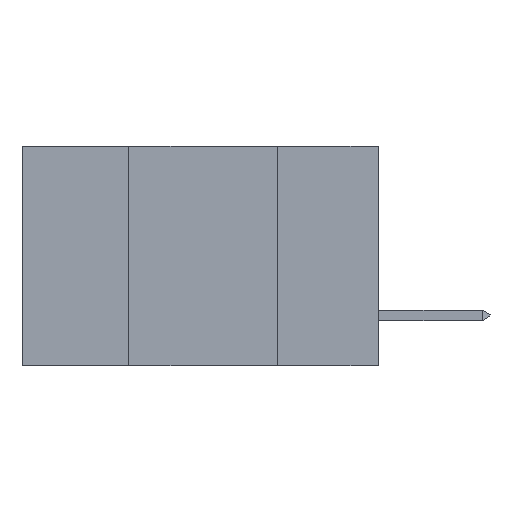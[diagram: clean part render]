
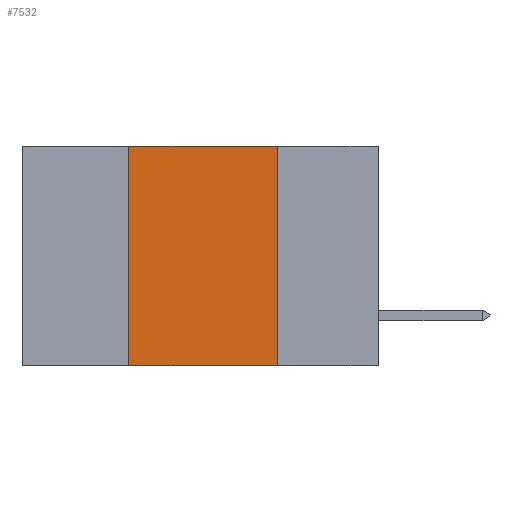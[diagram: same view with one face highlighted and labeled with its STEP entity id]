
A CAD part, left-side view. The second image highlights one B-rep face of the part: STEP entity #7532.
In plain terms, the highlighted planar face has unit normal (-1, 0, 0).
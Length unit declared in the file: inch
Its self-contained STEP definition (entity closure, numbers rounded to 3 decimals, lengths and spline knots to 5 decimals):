
#207 = VECTOR ( 'NONE', #2808, 39.37008 ) ;
#284 = FACE_OUTER_BOUND ( 'NONE', #3619, .T. ) ;
#699 = ORIENTED_EDGE ( 'NONE', *, *, #9616, .F. ) ;
#1013 = CARTESIAN_POINT ( 'NONE',  ( 0., 0.17, -0.37 ) ) ;
#1340 = CARTESIAN_POINT ( 'NONE',  ( 0., 0.6, 0. ) ) ;
#1343 = CARTESIAN_POINT ( 'NONE',  ( 0., 0.42, 0. ) ) ;
#2355 = VECTOR ( 'NONE', #12007, 39.37008 ) ;
#2480 = VERTEX_POINT ( 'NONE', #11958 ) ;
#2808 = DIRECTION ( 'NONE',  ( 0., 0., 1. ) ) ;
#2941 = LINE ( 'NONE', #12693, #8186 ) ;
#3619 = EDGE_LOOP ( 'NONE', ( #6959, #699, #4726, #6214 ) ) ;
#3783 = CARTESIAN_POINT ( 'NONE',  ( 0., 0.42, -0.37 ) ) ;
#4206 = VERTEX_POINT ( 'NONE', #1343 ) ;
#4246 = AXIS2_PLACEMENT_3D ( 'NONE', #1340, #12261, #10112 ) ;
#4351 = VERTEX_POINT ( 'NONE', #7938 ) ;
#4726 = ORIENTED_EDGE ( 'NONE', *, *, #5652, .F. ) ;
#5652 = EDGE_CURVE ( 'NONE', #12404, #4206, #10716, .T. ) ;
#6047 = PLANE ( 'NONE',  #4246 ) ;
#6214 = ORIENTED_EDGE ( 'NONE', *, *, #7336, .T. ) ;
#6959 = ORIENTED_EDGE ( 'NONE', *, *, #7340, .F. ) ;
#7336 = EDGE_CURVE ( 'NONE', #12404, #4351, #9989, .T. ) ;
#7340 = EDGE_CURVE ( 'NONE', #2480, #4351, #12789, .T. ) ;
#7532 = ADVANCED_FACE ( 'NONE', ( #284 ), #6047, .F. ) ;
#7938 = CARTESIAN_POINT ( 'NONE',  ( 0., 0.17, -0.37 ) ) ;
#8186 = VECTOR ( 'NONE', #11839, 39.37008 ) ;
#9616 = EDGE_CURVE ( 'NONE', #4206, #2480, #2941, .T. ) ;
#9989 = LINE ( 'NONE', #11877, #2355 ) ;
#10112 = DIRECTION ( 'NONE',  ( 0., 0., -1. ) ) ;
#10716 = LINE ( 'NONE', #3783, #207 ) ;
#11460 = CARTESIAN_POINT ( 'NONE',  ( 0., 0.42, -0.37 ) ) ;
#11751 = VECTOR ( 'NONE', #11942, 39.37008 ) ;
#11839 = DIRECTION ( 'NONE',  ( 0., -1., 0. ) ) ;
#11877 = CARTESIAN_POINT ( 'NONE',  ( 0., 0.6, -0.37 ) ) ;
#11942 = DIRECTION ( 'NONE',  ( 0., 0., -1. ) ) ;
#11958 = CARTESIAN_POINT ( 'NONE',  ( 0., 0.17, 0. ) ) ;
#12007 = DIRECTION ( 'NONE',  ( 0., -1., 0. ) ) ;
#12261 = DIRECTION ( 'NONE',  ( 1., 0., 0. ) ) ;
#12404 = VERTEX_POINT ( 'NONE', #11460 ) ;
#12693 = CARTESIAN_POINT ( 'NONE',  ( 0., 0.6, 0. ) ) ;
#12789 = LINE ( 'NONE', #1013, #11751 ) ;
